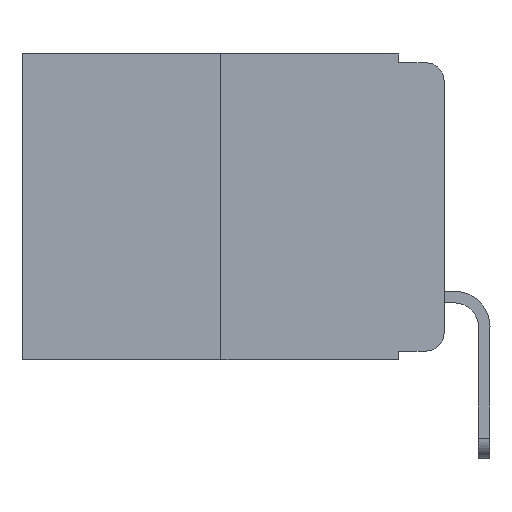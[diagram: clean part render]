
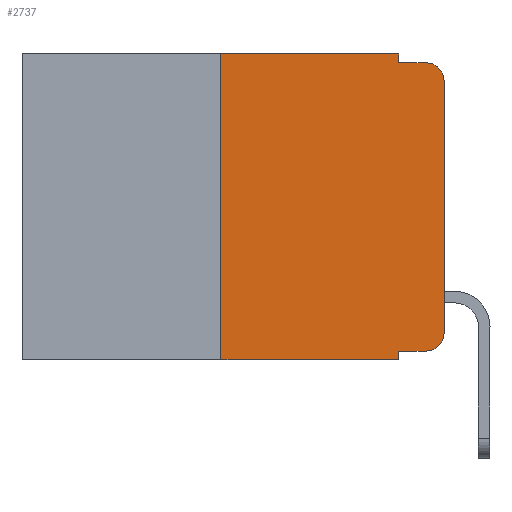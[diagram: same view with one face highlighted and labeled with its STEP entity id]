
A CAD part, left-side view. The second image highlights one B-rep face of the part: STEP entity #2737.
In plain terms, the highlighted planar face has unit normal (-1, 0, 0).
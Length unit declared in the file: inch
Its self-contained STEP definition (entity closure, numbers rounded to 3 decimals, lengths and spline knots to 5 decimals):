
#15 = CARTESIAN_POINT ( 'NONE',  ( 0., 0., -0.313 ) ) ;
#78 = PLANE ( 'NONE',  #3903 ) ;
#223 = CARTESIAN_POINT ( 'NONE',  ( 0., 0.051, -0.01 ) ) ;
#340 = DIRECTION ( 'NONE',  ( 0., -1., 0. ) ) ;
#373 = CARTESIAN_POINT ( 'NONE',  ( 0., 0.051, 0. ) ) ;
#432 = CARTESIAN_POINT ( 'NONE',  ( 0., 0.02, -0.01 ) ) ;
#652 = EDGE_CURVE ( 'NONE', #1996, #4473, #5537, .T. ) ;
#960 = VECTOR ( 'NONE', #11187, 39.37008 ) ;
#1208 = CARTESIAN_POINT ( 'NONE',  ( 0., 0., 0. ) ) ;
#1301 = VECTOR ( 'NONE', #7181, 39.37008 ) ;
#1469 = LINE ( 'NONE', #10040, #5544 ) ;
#1546 = CARTESIAN_POINT ( 'NONE',  ( 0., 0.051, 0. ) ) ;
#1996 = VERTEX_POINT ( 'NONE', #3709 ) ;
#2737 = ADVANCED_FACE ( 'NONE', ( #9748 ), #78, .F. ) ;
#3059 = EDGE_CURVE ( 'NONE', #4478, #5330, #10233, .T. ) ;
#3068 = CARTESIAN_POINT ( 'NONE',  ( 0., 0.473, -0.343 ) ) ;
#3129 = CARTESIAN_POINT ( 'NONE',  ( 0., 0., -0.03 ) ) ;
#3269 = VECTOR ( 'NONE', #3466, 39.37008 ) ;
#3313 = EDGE_CURVE ( 'NONE', #12632, #10612, #11343, .T. ) ;
#3368 = CARTESIAN_POINT ( 'NONE',  ( 0., 0.02, -0.333 ) ) ;
#3458 = VECTOR ( 'NONE', #7199, 39.37008 ) ;
#3466 = DIRECTION ( 'NONE',  ( 0., 0., -1. ) ) ;
#3500 = VERTEX_POINT ( 'NONE', #8262 ) ;
#3562 = CARTESIAN_POINT ( 'NONE',  ( 0., 0.051, -0.343 ) ) ;
#3579 = CARTESIAN_POINT ( 'NONE',  ( 0., 0.473, 0. ) ) ;
#3709 = CARTESIAN_POINT ( 'NONE',  ( 0., 0.25, -0.343 ) ) ;
#3903 = AXIS2_PLACEMENT_3D ( 'NONE', #12059, #7165, #8146 ) ;
#3909 = DIRECTION ( 'NONE',  ( -1., 0., 0. ) ) ;
#4157 = ORIENTED_EDGE ( 'NONE', *, *, #13042, .T. ) ;
#4247 = CARTESIAN_POINT ( 'NONE',  ( 0., 0.051, -0.333 ) ) ;
#4287 = ORIENTED_EDGE ( 'NONE', *, *, #8319, .F. ) ;
#4473 = VERTEX_POINT ( 'NONE', #9132 ) ;
#4478 = VERTEX_POINT ( 'NONE', #3129 ) ;
#4557 = VERTEX_POINT ( 'NONE', #3368 ) ;
#4596 = DIRECTION ( 'NONE',  ( 0., -1., 0. ) ) ;
#4794 = EDGE_CURVE ( 'NONE', #4557, #11526, #8184, .T. ) ;
#4894 = LINE ( 'NONE', #3068, #3458 ) ;
#5178 = EDGE_CURVE ( 'NONE', #3500, #5330, #7804, .T. ) ;
#5194 = ORIENTED_EDGE ( 'NONE', *, *, #5581, .T. ) ;
#5330 = VERTEX_POINT ( 'NONE', #432 ) ;
#5537 = LINE ( 'NONE', #11230, #1301 ) ;
#5544 = VECTOR ( 'NONE', #11161, 39.37008 ) ;
#5581 = EDGE_CURVE ( 'NONE', #12632, #4557, #5585, .T. ) ;
#5585 = LINE ( 'NONE', #8117, #8923 ) ;
#6209 = ORIENTED_EDGE ( 'NONE', *, *, #5178, .F. ) ;
#6631 = DIRECTION ( 'NONE',  ( 0., 0., -1. ) ) ;
#6671 = CARTESIAN_POINT ( 'NONE',  ( 0., 0.02, -0.313 ) ) ;
#7042 = ORIENTED_EDGE ( 'NONE', *, *, #652, .F. ) ;
#7165 = DIRECTION ( 'NONE',  ( 1., 0., 0. ) ) ;
#7181 = DIRECTION ( 'NONE',  ( 0., 0., 1. ) ) ;
#7199 = DIRECTION ( 'NONE',  ( 0., -1., 0. ) ) ;
#7804 = LINE ( 'NONE', #223, #10822 ) ;
#7873 = CARTESIAN_POINT ( 'NONE',  ( 0., 0.02, -0.03 ) ) ;
#7877 = AXIS2_PLACEMENT_3D ( 'NONE', #7873, #3909, #10991 ) ;
#8117 = CARTESIAN_POINT ( 'NONE',  ( 0., 0.051, -0.333 ) ) ;
#8146 = DIRECTION ( 'NONE',  ( 0., 0., -1. ) ) ;
#8184 = CIRCLE ( 'NONE', #9407, 0.02 ) ;
#8262 = CARTESIAN_POINT ( 'NONE',  ( 0., 0.051, -0.01 ) ) ;
#8319 = EDGE_CURVE ( 'NONE', #12038, #3500, #1469, .T. ) ;
#8821 = ORIENTED_EDGE ( 'NONE', *, *, #12723, .F. ) ;
#8923 = VECTOR ( 'NONE', #12150, 39.37008 ) ;
#9096 = ORIENTED_EDGE ( 'NONE', *, *, #3313, .F. ) ;
#9132 = CARTESIAN_POINT ( 'NONE',  ( 0., 0.25, 0. ) ) ;
#9407 = AXIS2_PLACEMENT_3D ( 'NONE', #6671, #12701, #6631 ) ;
#9748 = FACE_OUTER_BOUND ( 'NONE', #11239, .T. ) ;
#10040 = CARTESIAN_POINT ( 'NONE',  ( 0., 0.051, 0. ) ) ;
#10233 = CIRCLE ( 'NONE', #7877, 0.02 ) ;
#10298 = ORIENTED_EDGE ( 'NONE', *, *, #3059, .T. ) ;
#10612 = VERTEX_POINT ( 'NONE', #3562 ) ;
#10774 = ORIENTED_EDGE ( 'NONE', *, *, #12416, .T. ) ;
#10822 = VECTOR ( 'NONE', #340, 39.37008 ) ;
#10942 = ORIENTED_EDGE ( 'NONE', *, *, #4794, .T. ) ;
#10991 = DIRECTION ( 'NONE',  ( 0., 0., -1. ) ) ;
#11161 = DIRECTION ( 'NONE',  ( 0., 0., -1. ) ) ;
#11187 = DIRECTION ( 'NONE',  ( 0., 0., 1. ) ) ;
#11230 = CARTESIAN_POINT ( 'NONE',  ( 0., 0.25, 0. ) ) ;
#11239 = EDGE_LOOP ( 'NONE', ( #4157, #10298, #6209, #4287, #8821, #7042, #10774, #9096, #5194, #10942 ) ) ;
#11343 = LINE ( 'NONE', #373, #3269 ) ;
#11526 = VERTEX_POINT ( 'NONE', #15 ) ;
#11684 = LINE ( 'NONE', #1208, #960 ) ;
#12038 = VERTEX_POINT ( 'NONE', #1546 ) ;
#12059 = CARTESIAN_POINT ( 'NONE',  ( 0., 0.473, 0. ) ) ;
#12150 = DIRECTION ( 'NONE',  ( 0., -1., 0. ) ) ;
#12416 = EDGE_CURVE ( 'NONE', #1996, #10612, #4894, .T. ) ;
#12625 = VECTOR ( 'NONE', #4596, 39.37008 ) ;
#12632 = VERTEX_POINT ( 'NONE', #4247 ) ;
#12701 = DIRECTION ( 'NONE',  ( -1., 0., 0. ) ) ;
#12723 = EDGE_CURVE ( 'NONE', #4473, #12038, #12791, .T. ) ;
#12791 = LINE ( 'NONE', #3579, #12625 ) ;
#13042 = EDGE_CURVE ( 'NONE', #11526, #4478, #11684, .T. ) ;
